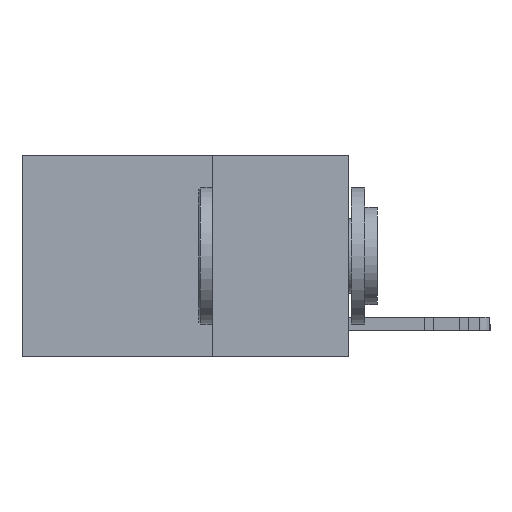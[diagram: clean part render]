
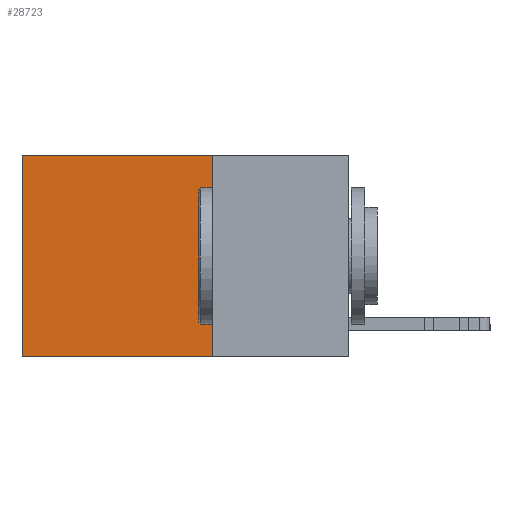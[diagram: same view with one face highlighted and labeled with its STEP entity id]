
A CAD part, left-side view. The second image highlights one B-rep face of the part: STEP entity #28723.
In plain terms, the highlighted planar face has unit normal (-1, 0, 0).
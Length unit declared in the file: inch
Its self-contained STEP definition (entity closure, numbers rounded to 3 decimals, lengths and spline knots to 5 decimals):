
#545 = ORIENTED_EDGE ( 'NONE', *, *, #14586, .T. ) ;
#1274 = DIRECTION ( 'NONE',  ( 1., 0., 0. ) ) ;
#1376 = VERTEX_POINT ( 'NONE', #9021 ) ;
#1479 = CARTESIAN_POINT ( 'NONE',  ( 0.2625, 0.6, 0. ) ) ;
#2341 = VERTEX_POINT ( 'NONE', #11203 ) ;
#2830 = ORIENTED_EDGE ( 'NONE', *, *, #21596, .T. ) ;
#3155 = LINE ( 'NONE', #25103, #19911 ) ;
#3755 = CARTESIAN_POINT ( 'NONE',  ( 0.2625, 0.25, -0.37 ) ) ;
#4301 = CARTESIAN_POINT ( 'NONE',  ( 0.2625, 0.25, 0. ) ) ;
#4571 = AXIS2_PLACEMENT_3D ( 'NONE', #12815, #1274, #10329 ) ;
#5479 = EDGE_CURVE ( 'NONE', #28206, #1376, #17300, .T. ) ;
#7074 = CARTESIAN_POINT ( 'NONE',  ( 0.2625, 0.25, 0. ) ) ;
#7624 = VERTEX_POINT ( 'NONE', #1479 ) ;
#8729 = VECTOR ( 'NONE', #16856, 39.37008 ) ;
#8855 = VECTOR ( 'NONE', #16031, 39.37008 ) ;
#9021 = CARTESIAN_POINT ( 'NONE',  ( 0.2625, 0.6, -0.37 ) ) ;
#9976 = DIRECTION ( 'NONE',  ( 0., 0., -1. ) ) ;
#10014 = PLANE ( 'NONE',  #4571 ) ;
#10162 = FACE_OUTER_BOUND ( 'NONE', #23359, .T. ) ;
#10329 = DIRECTION ( 'NONE',  ( 0., 0., -1. ) ) ;
#11203 = CARTESIAN_POINT ( 'NONE',  ( 0.2625, 0.25, 0. ) ) ;
#12815 = CARTESIAN_POINT ( 'NONE',  ( 0.2625, 0.25, 0. ) ) ;
#12868 = VECTOR ( 'NONE', #22136, 39.37008 ) ;
#13829 = LINE ( 'NONE', #7074, #8855 ) ;
#14586 = EDGE_CURVE ( 'NONE', #2341, #7624, #28996, .T. ) ;
#14890 = ORIENTED_EDGE ( 'NONE', *, *, #24900, .F. ) ;
#16031 = DIRECTION ( 'NONE',  ( 0., 0., -1. ) ) ;
#16856 = DIRECTION ( 'NONE',  ( 0., 1., 0. ) ) ;
#17300 = LINE ( 'NONE', #3755, #8729 ) ;
#19911 = VECTOR ( 'NONE', #9976, 39.37008 ) ;
#21596 = EDGE_CURVE ( 'NONE', #7624, #1376, #3155, .T. ) ;
#21959 = CARTESIAN_POINT ( 'NONE',  ( 0.2625, 0.25, -0.37 ) ) ;
#22136 = DIRECTION ( 'NONE',  ( 0., 1., 0. ) ) ;
#22824 = ORIENTED_EDGE ( 'NONE', *, *, #5479, .F. ) ;
#23359 = EDGE_LOOP ( 'NONE', ( #2830, #22824, #14890, #545 ) ) ;
#24900 = EDGE_CURVE ( 'NONE', #2341, #28206, #13829, .T. ) ;
#25103 = CARTESIAN_POINT ( 'NONE',  ( 0.2625, 0.6, 0. ) ) ;
#28206 = VERTEX_POINT ( 'NONE', #21959 ) ;
#28723 = ADVANCED_FACE ( 'NONE', ( #10162 ), #10014, .F. ) ;
#28996 = LINE ( 'NONE', #4301, #12868 ) ;
